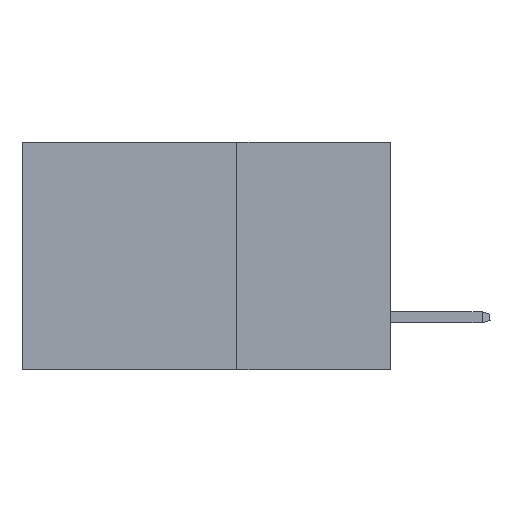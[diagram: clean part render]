
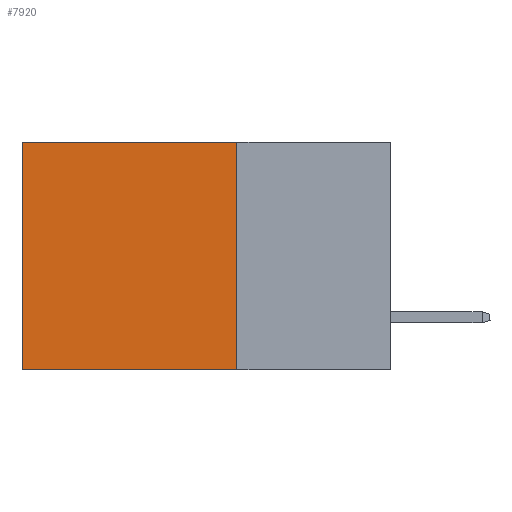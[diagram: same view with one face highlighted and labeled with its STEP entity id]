
A CAD part, left-side view. The second image highlights one B-rep face of the part: STEP entity #7920.
In plain terms, the highlighted planar face has unit normal (-1, 0, 0).
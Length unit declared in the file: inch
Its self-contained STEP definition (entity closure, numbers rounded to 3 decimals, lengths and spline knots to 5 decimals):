
#1333 = DIRECTION ( 'NONE',  ( 0., 0., -1. ) ) ;
#1588 = CARTESIAN_POINT ( 'NONE',  ( 0.2875, 0.6, 0. ) ) ;
#1736 = CARTESIAN_POINT ( 'NONE',  ( 0.2875, 0.25, 0. ) ) ;
#1993 = CARTESIAN_POINT ( 'NONE',  ( 0.2875, 0.25, -0.37 ) ) ;
#2092 = CARTESIAN_POINT ( 'NONE',  ( 0.2875, 0.25, 0. ) ) ;
#3356 = EDGE_CURVE ( 'NONE', #12495, #13959, #18219, .T. ) ;
#3466 = EDGE_CURVE ( 'NONE', #12495, #6499, #16927, .T. ) ;
#3984 = LINE ( 'NONE', #10957, #4738 ) ;
#4035 = VECTOR ( 'NONE', #21014, 39.37008 ) ;
#4644 = CARTESIAN_POINT ( 'NONE',  ( 0.2875, 0.25, 0. ) ) ;
#4685 = VECTOR ( 'NONE', #17693, 39.37008 ) ;
#4738 = VECTOR ( 'NONE', #15865, 39.37008 ) ;
#5541 = ORIENTED_EDGE ( 'NONE', *, *, #14913, .F. ) ;
#5580 = LINE ( 'NONE', #1588, #4035 ) ;
#6499 = VERTEX_POINT ( 'NONE', #19669 ) ;
#7566 = ORIENTED_EDGE ( 'NONE', *, *, #3466, .T. ) ;
#7920 = ADVANCED_FACE ( 'NONE', ( #20052 ), #20061, .F. ) ;
#8039 = ORIENTED_EDGE ( 'NONE', *, *, #3356, .F. ) ;
#8419 = ORIENTED_EDGE ( 'NONE', *, *, #19176, .T. ) ;
#10957 = CARTESIAN_POINT ( 'NONE',  ( 0.2875, 0.25, -0.37 ) ) ;
#12175 = CARTESIAN_POINT ( 'NONE',  ( 0.2875, 0.6, -0.37 ) ) ;
#12495 = VERTEX_POINT ( 'NONE', #1736 ) ;
#13549 = VECTOR ( 'NONE', #20225, 39.37008 ) ;
#13674 = VERTEX_POINT ( 'NONE', #12175 ) ;
#13959 = VERTEX_POINT ( 'NONE', #1993 ) ;
#14135 = AXIS2_PLACEMENT_3D ( 'NONE', #16893, #18751, #1333 ) ;
#14913 = EDGE_CURVE ( 'NONE', #13959, #13674, #3984, .T. ) ;
#15865 = DIRECTION ( 'NONE',  ( 0., 1., 0. ) ) ;
#16893 = CARTESIAN_POINT ( 'NONE',  ( 0.2875, 0.25, 0. ) ) ;
#16927 = LINE ( 'NONE', #2092, #13549 ) ;
#17693 = DIRECTION ( 'NONE',  ( 0., 0., -1. ) ) ;
#17707 = EDGE_LOOP ( 'NONE', ( #8419, #5541, #8039, #7566 ) ) ;
#18219 = LINE ( 'NONE', #4644, #4685 ) ;
#18751 = DIRECTION ( 'NONE',  ( 1., 0., 0. ) ) ;
#19176 = EDGE_CURVE ( 'NONE', #6499, #13674, #5580, .T. ) ;
#19669 = CARTESIAN_POINT ( 'NONE',  ( 0.2875, 0.6, 0. ) ) ;
#20052 = FACE_OUTER_BOUND ( 'NONE', #17707, .T. ) ;
#20061 = PLANE ( 'NONE',  #14135 ) ;
#20225 = DIRECTION ( 'NONE',  ( 0., 1., 0. ) ) ;
#21014 = DIRECTION ( 'NONE',  ( 0., 0., -1. ) ) ;
